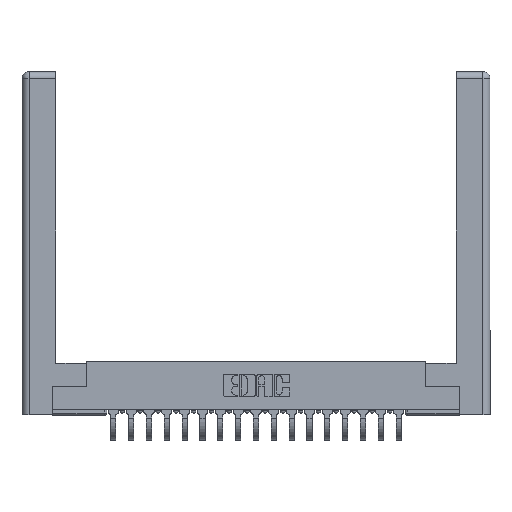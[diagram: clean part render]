
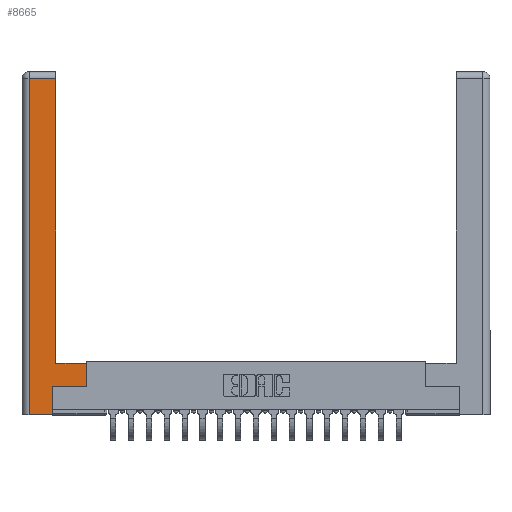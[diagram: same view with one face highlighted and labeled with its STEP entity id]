
A CAD part, top view. The second image highlights one B-rep face of the part: STEP entity #8665.
In plain terms, the highlighted planar face has unit normal (0, 0, 1).
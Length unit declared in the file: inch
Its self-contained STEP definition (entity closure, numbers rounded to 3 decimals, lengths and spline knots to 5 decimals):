
#153 = VECTOR ( 'NONE', #6334, 39.37008 ) ;
#389 = DIRECTION ( 'NONE',  ( -1., 0., 0. ) ) ;
#486 = EDGE_CURVE ( 'NONE', #1190, #4738, #7728, .T. ) ;
#754 = VECTOR ( 'NONE', #7690, 39.37008 ) ;
#969 = ORIENTED_EDGE ( 'NONE', *, *, #18181, .T. ) ;
#1093 = ORIENTED_EDGE ( 'NONE', *, *, #12960, .T. ) ;
#1190 = VERTEX_POINT ( 'NONE', #11980 ) ;
#1424 = VERTEX_POINT ( 'NONE', #12757 ) ;
#1544 = ORIENTED_EDGE ( 'NONE', *, *, #21864, .T. ) ;
#1594 = VECTOR ( 'NONE', #10417, 39.37008 ) ;
#1920 = EDGE_CURVE ( 'NONE', #1424, #8180, #21510, .T. ) ;
#2041 = CARTESIAN_POINT ( 'NONE',  ( 0.265, 0.245, 0. ) ) ;
#2412 = EDGE_CURVE ( 'NONE', #8180, #18489, #4412, .T. ) ;
#2464 = CARTESIAN_POINT ( 'NONE',  ( 0.0615, 2.94, 0. ) ) ;
#2524 = FACE_OUTER_BOUND ( 'NONE', #9131, .T. ) ;
#2599 = CARTESIAN_POINT ( 'NONE',  ( 0.295, 0.45, 0. ) ) ;
#2653 = VERTEX_POINT ( 'NONE', #2464 ) ;
#2953 = ORIENTED_EDGE ( 'NONE', *, *, #6032, .T. ) ;
#4221 = ORIENTED_EDGE ( 'NONE', *, *, #4632, .T. ) ;
#4242 = CARTESIAN_POINT ( 'NONE',  ( 0.565, 0.45, 0. ) ) ;
#4272 = CARTESIAN_POINT ( 'NONE',  ( 0.295, 2.94, 0. ) ) ;
#4401 = LINE ( 'NONE', #21888, #11893 ) ;
#4412 = LINE ( 'NONE', #11315, #153 ) ;
#4624 = DIRECTION ( 'NONE',  ( 1., 0., 0. ) ) ;
#4632 = EDGE_CURVE ( 'NONE', #18489, #17526, #5316, .T. ) ;
#4738 = VERTEX_POINT ( 'NONE', #2041 ) ;
#5316 = LINE ( 'NONE', #8388, #754 ) ;
#6032 = EDGE_CURVE ( 'NONE', #4738, #1424, #9616, .T. ) ;
#6160 = DIRECTION ( 'NONE',  ( 0., 1., 0. ) ) ;
#6334 = DIRECTION ( 'NONE',  ( -1., 0., 0. ) ) ;
#6914 = CARTESIAN_POINT ( 'NONE',  ( 0.0615, 2.94, 0. ) ) ;
#7609 = DIRECTION ( 'NONE',  ( 0., 1., 0. ) ) ;
#7666 = VECTOR ( 'NONE', #6160, 39.37008 ) ;
#7690 = DIRECTION ( 'NONE',  ( 0., 1., 0. ) ) ;
#7728 = LINE ( 'NONE', #12821, #11332 ) ;
#8180 = VERTEX_POINT ( 'NONE', #12075 ) ;
#8388 = CARTESIAN_POINT ( 'NONE',  ( 0.295, 3., 0. ) ) ;
#8665 = ADVANCED_FACE ( 'NONE', ( #2524 ), #21375, .F. ) ;
#8930 = CARTESIAN_POINT ( 'NONE',  ( 0.0615, 0., 0. ) ) ;
#9131 = EDGE_LOOP ( 'NONE', ( #4221, #1093, #969, #1544, #12139, #2953, #12865, #15153 ) ) ;
#9616 = LINE ( 'NONE', #11649, #15699 ) ;
#10417 = DIRECTION ( 'NONE',  ( -1., 0., 0. ) ) ;
#10904 = CARTESIAN_POINT ( 'NONE',  ( 0., 0., 0. ) ) ;
#11315 = CARTESIAN_POINT ( 'NONE',  ( 0.295, 0.45, 0. ) ) ;
#11332 = VECTOR ( 'NONE', #7609, 39.37008 ) ;
#11649 = CARTESIAN_POINT ( 'NONE',  ( 0.565, 0.245, 0. ) ) ;
#11893 = VECTOR ( 'NONE', #4624, 39.37008 ) ;
#11980 = CARTESIAN_POINT ( 'NONE',  ( 0.265, 0., 0. ) ) ;
#12075 = CARTESIAN_POINT ( 'NONE',  ( 0.565, 0.45, 0. ) ) ;
#12139 = ORIENTED_EDGE ( 'NONE', *, *, #486, .T. ) ;
#12757 = CARTESIAN_POINT ( 'NONE',  ( 0.565, 0.245, 0. ) ) ;
#12821 = CARTESIAN_POINT ( 'NONE',  ( 0.265, 0.245, 0. ) ) ;
#12865 = ORIENTED_EDGE ( 'NONE', *, *, #1920, .T. ) ;
#12960 = EDGE_CURVE ( 'NONE', #17526, #2653, #17308, .T. ) ;
#13488 = CARTESIAN_POINT ( 'NONE',  ( 0.0615, 0., 0. ) ) ;
#15153 = ORIENTED_EDGE ( 'NONE', *, *, #2412, .T. ) ;
#15513 = LINE ( 'NONE', #13488, #21032 ) ;
#15699 = VECTOR ( 'NONE', #22014, 39.37008 ) ;
#15981 = AXIS2_PLACEMENT_3D ( 'NONE', #10904, #19470, #389 ) ;
#17034 = VERTEX_POINT ( 'NONE', #8930 ) ;
#17308 = LINE ( 'NONE', #6914, #1594 ) ;
#17526 = VERTEX_POINT ( 'NONE', #4272 ) ;
#18181 = EDGE_CURVE ( 'NONE', #2653, #17034, #15513, .T. ) ;
#18489 = VERTEX_POINT ( 'NONE', #2599 ) ;
#19470 = DIRECTION ( 'NONE',  ( 0., 0., -1. ) ) ;
#21032 = VECTOR ( 'NONE', #22161, 39.37008 ) ;
#21375 = PLANE ( 'NONE',  #15981 ) ;
#21510 = LINE ( 'NONE', #4242, #7666 ) ;
#21864 = EDGE_CURVE ( 'NONE', #17034, #1190, #4401, .T. ) ;
#21888 = CARTESIAN_POINT ( 'NONE',  ( 0.265, 0., 0. ) ) ;
#22014 = DIRECTION ( 'NONE',  ( 1., 0., 0. ) ) ;
#22161 = DIRECTION ( 'NONE',  ( 0., -1., 0. ) ) ;
